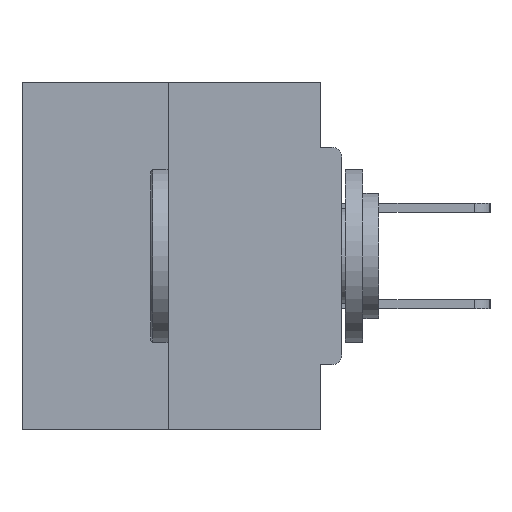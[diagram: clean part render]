
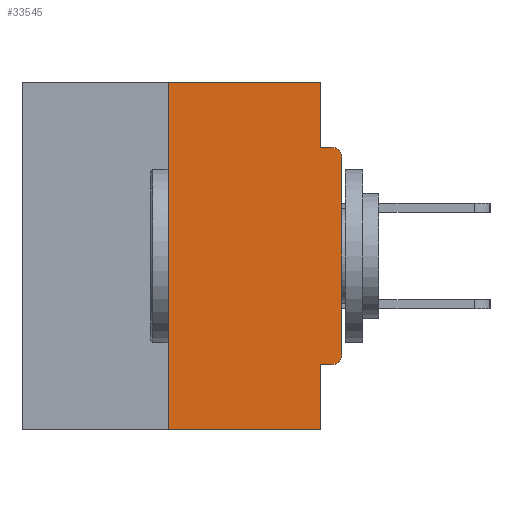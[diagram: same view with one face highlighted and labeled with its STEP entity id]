
A CAD part, left-side view. The second image highlights one B-rep face of the part: STEP entity #33545.
In plain terms, the highlighted planar face has unit normal (-1, 0, 0).
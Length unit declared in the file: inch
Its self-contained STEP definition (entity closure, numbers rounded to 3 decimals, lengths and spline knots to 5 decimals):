
#684 = LINE ( 'NONE', #30311, #35304 ) ;
#1015 = CARTESIAN_POINT ( 'NONE',  ( 0., 0., -0.1085 ) ) ;
#1242 = VECTOR ( 'NONE', #19865, 39.37008 ) ;
#1481 = CARTESIAN_POINT ( 'NONE',  ( 0., 0., -0.3915 ) ) ;
#1601 = CARTESIAN_POINT ( 'NONE',  ( 0., 0.015, -0.3915 ) ) ;
#2022 = DIRECTION ( 'NONE',  ( 0., 0., -1. ) ) ;
#2091 = DIRECTION ( 'NONE',  ( 0., 0., -1. ) ) ;
#2158 = EDGE_CURVE ( 'NONE', #34007, #10691, #30401, .T. ) ;
#2440 = ORIENTED_EDGE ( 'NONE', *, *, #6152, .F. ) ;
#2453 = CARTESIAN_POINT ( 'NONE',  ( 0., 0.25, 0. ) ) ;
#2547 = VERTEX_POINT ( 'NONE', #1015 ) ;
#3452 = CARTESIAN_POINT ( 'NONE',  ( 0., 0.46, 0. ) ) ;
#4786 = EDGE_CURVE ( 'NONE', #5796, #30951, #15176, .T. ) ;
#5796 = VERTEX_POINT ( 'NONE', #31595 ) ;
#5871 = LINE ( 'NONE', #33909, #35470 ) ;
#6152 = EDGE_CURVE ( 'NONE', #34007, #18372, #684, .T. ) ;
#6810 = ORIENTED_EDGE ( 'NONE', *, *, #2158, .T. ) ;
#6875 = LINE ( 'NONE', #31227, #21400 ) ;
#6973 = FACE_OUTER_BOUND ( 'NONE', #14991, .T. ) ;
#7259 = DIRECTION ( 'NONE',  ( 0., 0., 1. ) ) ;
#7352 = DIRECTION ( 'NONE',  ( 0., 0., -1. ) ) ;
#7598 = CARTESIAN_POINT ( 'NONE',  ( 0., 0.031, -0.5 ) ) ;
#8045 = CARTESIAN_POINT ( 'NONE',  ( 0., 0.031, -0.0935 ) ) ;
#8386 = VECTOR ( 'NONE', #9961, 39.37008 ) ;
#8407 = AXIS2_PLACEMENT_3D ( 'NONE', #30923, #37049, #2022 ) ;
#8773 = CARTESIAN_POINT ( 'NONE',  ( 0., 0.25, -0.5 ) ) ;
#8942 = PLANE ( 'NONE',  #12031 ) ;
#9132 = LINE ( 'NONE', #34235, #28717 ) ;
#9481 = CARTESIAN_POINT ( 'NONE',  ( 0., 0.015, -0.0935 ) ) ;
#9565 = ORIENTED_EDGE ( 'NONE', *, *, #12951, .F. ) ;
#9649 = EDGE_CURVE ( 'NONE', #31053, #31956, #6875, .T. ) ;
#9672 = VERTEX_POINT ( 'NONE', #22548 ) ;
#9961 = DIRECTION ( 'NONE',  ( 0., -1., 0. ) ) ;
#10123 = CARTESIAN_POINT ( 'NONE',  ( 0., 0.46, 0. ) ) ;
#10267 = DIRECTION ( 'NONE',  ( 0., 0., -1. ) ) ;
#10691 = VERTEX_POINT ( 'NONE', #34161 ) ;
#12031 = AXIS2_PLACEMENT_3D ( 'NONE', #3452, #35027, #17922 ) ;
#12925 = CARTESIAN_POINT ( 'NONE',  ( 0., 0.46, -0.5 ) ) ;
#12951 = EDGE_CURVE ( 'NONE', #9672, #10691, #21291, .T. ) ;
#13163 = DIRECTION ( 'NONE',  ( -1., 0., 0. ) ) ;
#13269 = VECTOR ( 'NONE', #16050, 39.37008 ) ;
#13362 = ORIENTED_EDGE ( 'NONE', *, *, #24764, .F. ) ;
#13544 = VECTOR ( 'NONE', #7352, 39.37008 ) ;
#13642 = DIRECTION ( 'NONE',  ( 0., 1., 0. ) ) ;
#13695 = AXIS2_PLACEMENT_3D ( 'NONE', #1601, #13163, #10267 ) ;
#14991 = EDGE_LOOP ( 'NONE', ( #20665, #2440, #6810, #9565, #21038, #19222, #17083, #15800, #13362, #28044 ) ) ;
#15176 = CIRCLE ( 'NONE', #13695, 0.015 ) ;
#15800 = ORIENTED_EDGE ( 'NONE', *, *, #35922, .T. ) ;
#16050 = DIRECTION ( 'NONE',  ( 0., -1., 0. ) ) ;
#17083 = ORIENTED_EDGE ( 'NONE', *, *, #20496, .T. ) ;
#17447 = LINE ( 'NONE', #18453, #8386 ) ;
#17922 = DIRECTION ( 'NONE',  ( 0., 0., -1. ) ) ;
#18372 = VERTEX_POINT ( 'NONE', #2453 ) ;
#18453 = CARTESIAN_POINT ( 'NONE',  ( 0., 0., -0.0935 ) ) ;
#19222 = ORIENTED_EDGE ( 'NONE', *, *, #4786, .T. ) ;
#19865 = DIRECTION ( 'NONE',  ( 0., -1., 0. ) ) ;
#20496 = EDGE_CURVE ( 'NONE', #30951, #2547, #9132, .T. ) ;
#20665 = ORIENTED_EDGE ( 'NONE', *, *, #34187, .F. ) ;
#21038 = ORIENTED_EDGE ( 'NONE', *, *, #28883, .F. ) ;
#21291 = LINE ( 'NONE', #7598, #13544 ) ;
#21400 = VECTOR ( 'NONE', #2091, 39.37008 ) ;
#22548 = CARTESIAN_POINT ( 'NONE',  ( 0., 0.031, -0.4065 ) ) ;
#22823 = CARTESIAN_POINT ( 'NONE',  ( 0., 0.031, 0. ) ) ;
#24060 = VERTEX_POINT ( 'NONE', #9481 ) ;
#24764 = EDGE_CURVE ( 'NONE', #31956, #24060, #17447, .T. ) ;
#24971 = CIRCLE ( 'NONE', #8407, 0.015 ) ;
#25683 = DIRECTION ( 'NONE',  ( 0., 0., 1. ) ) ;
#28044 = ORIENTED_EDGE ( 'NONE', *, *, #9649, .F. ) ;
#28717 = VECTOR ( 'NONE', #25683, 39.37008 ) ;
#28883 = EDGE_CURVE ( 'NONE', #5796, #9672, #5871, .T. ) ;
#30311 = CARTESIAN_POINT ( 'NONE',  ( 0., 0.25, 0. ) ) ;
#30401 = LINE ( 'NONE', #12925, #1242 ) ;
#30923 = CARTESIAN_POINT ( 'NONE',  ( 0., 0.015, -0.1085 ) ) ;
#30951 = VERTEX_POINT ( 'NONE', #1481 ) ;
#31053 = VERTEX_POINT ( 'NONE', #22823 ) ;
#31227 = CARTESIAN_POINT ( 'NONE',  ( 0., 0.031, 0. ) ) ;
#31595 = CARTESIAN_POINT ( 'NONE',  ( 0., 0.015, -0.4065 ) ) ;
#31956 = VERTEX_POINT ( 'NONE', #8045 ) ;
#33545 = ADVANCED_FACE ( 'NONE', ( #6973 ), #8942, .F. ) ;
#33909 = CARTESIAN_POINT ( 'NONE',  ( 0., 0., -0.4065 ) ) ;
#34007 = VERTEX_POINT ( 'NONE', #8773 ) ;
#34161 = CARTESIAN_POINT ( 'NONE',  ( 0., 0.031, -0.5 ) ) ;
#34187 = EDGE_CURVE ( 'NONE', #18372, #31053, #37470, .T. ) ;
#34235 = CARTESIAN_POINT ( 'NONE',  ( 0., 0., 0. ) ) ;
#35027 = DIRECTION ( 'NONE',  ( 1., 0., 0. ) ) ;
#35304 = VECTOR ( 'NONE', #7259, 39.37008 ) ;
#35470 = VECTOR ( 'NONE', #13642, 39.37008 ) ;
#35922 = EDGE_CURVE ( 'NONE', #2547, #24060, #24971, .T. ) ;
#37049 = DIRECTION ( 'NONE',  ( -1., 0., 0. ) ) ;
#37470 = LINE ( 'NONE', #10123, #13269 ) ;
